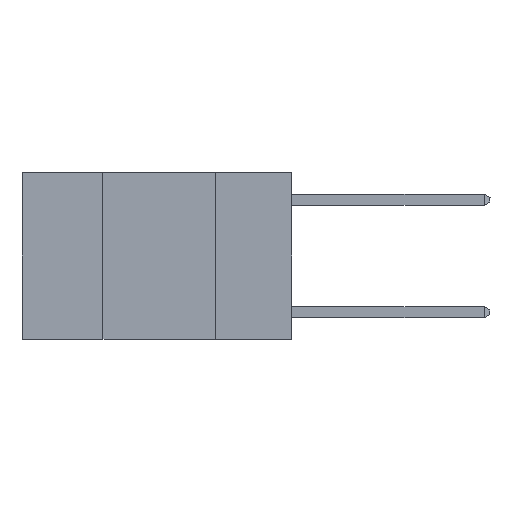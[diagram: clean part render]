
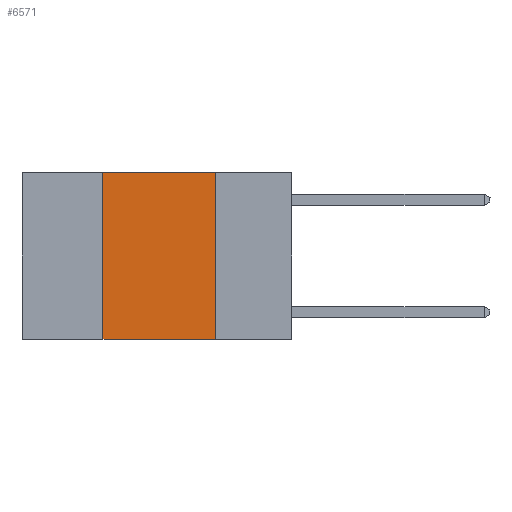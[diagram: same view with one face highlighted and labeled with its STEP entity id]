
A CAD part, left-side view. The second image highlights one B-rep face of the part: STEP entity #6571.
In plain terms, the highlighted planar face has unit normal (-1, 0, 0).
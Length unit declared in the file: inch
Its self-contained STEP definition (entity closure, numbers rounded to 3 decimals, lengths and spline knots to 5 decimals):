
#767 = EDGE_CURVE ( 'NONE', #3539, #6102, #1992, .T. ) ;
#1259 = EDGE_LOOP ( 'NONE', ( #6044, #7261, #6596, #7849 ) ) ;
#1333 = DIRECTION ( 'NONE',  ( 1., 0., 0. ) ) ;
#1693 = LINE ( 'NONE', #7606, #3840 ) ;
#1992 = LINE ( 'NONE', #9216, #3672 ) ;
#2010 = VECTOR ( 'NONE', #3251, 39.37008 ) ;
#2110 = DIRECTION ( 'NONE',  ( 0., 0., -1. ) ) ;
#2164 = FACE_OUTER_BOUND ( 'NONE', #1259, .T. ) ;
#2172 = CARTESIAN_POINT ( 'NONE',  ( 0., 0.42, 0. ) ) ;
#2297 = VECTOR ( 'NONE', #2110, 39.37008 ) ;
#2316 = VERTEX_POINT ( 'NONE', #6360 ) ;
#2795 = LINE ( 'NONE', #8603, #2297 ) ;
#2808 = CARTESIAN_POINT ( 'NONE',  ( 0., 0.17, 0. ) ) ;
#3251 = DIRECTION ( 'NONE',  ( 0., -1., 0. ) ) ;
#3460 = CARTESIAN_POINT ( 'NONE',  ( 0., 0.6, 0. ) ) ;
#3539 = VERTEX_POINT ( 'NONE', #6220 ) ;
#3672 = VECTOR ( 'NONE', #7066, 39.37008 ) ;
#3840 = VECTOR ( 'NONE', #8380, 39.37008 ) ;
#3961 = LINE ( 'NONE', #6869, #2010 ) ;
#4842 = EDGE_CURVE ( 'NONE', #3539, #2316, #1693, .T. ) ;
#5000 = EDGE_CURVE ( 'NONE', #9243, #2316, #2795, .T. ) ;
#5137 = DIRECTION ( 'NONE',  ( 0., 0., -1. ) ) ;
#5181 = AXIS2_PLACEMENT_3D ( 'NONE', #3460, #1333, #5137 ) ;
#5865 = EDGE_CURVE ( 'NONE', #6102, #9243, #3961, .T. ) ;
#6044 = ORIENTED_EDGE ( 'NONE', *, *, #5000, .F. ) ;
#6102 = VERTEX_POINT ( 'NONE', #2172 ) ;
#6220 = CARTESIAN_POINT ( 'NONE',  ( 0., 0.42, -0.37 ) ) ;
#6360 = CARTESIAN_POINT ( 'NONE',  ( 0., 0.17, -0.37 ) ) ;
#6571 = ADVANCED_FACE ( 'NONE', ( #2164 ), #7176, .F. ) ;
#6596 = ORIENTED_EDGE ( 'NONE', *, *, #767, .F. ) ;
#6869 = CARTESIAN_POINT ( 'NONE',  ( 0., 0.6, 0. ) ) ;
#7066 = DIRECTION ( 'NONE',  ( 0., 0., 1. ) ) ;
#7176 = PLANE ( 'NONE',  #5181 ) ;
#7261 = ORIENTED_EDGE ( 'NONE', *, *, #5865, .F. ) ;
#7606 = CARTESIAN_POINT ( 'NONE',  ( 0., 0.6, -0.37 ) ) ;
#7849 = ORIENTED_EDGE ( 'NONE', *, *, #4842, .T. ) ;
#8380 = DIRECTION ( 'NONE',  ( 0., -1., 0. ) ) ;
#8603 = CARTESIAN_POINT ( 'NONE',  ( 0., 0.17, 0. ) ) ;
#9216 = CARTESIAN_POINT ( 'NONE',  ( 0., 0.42, 0. ) ) ;
#9243 = VERTEX_POINT ( 'NONE', #2808 ) ;
